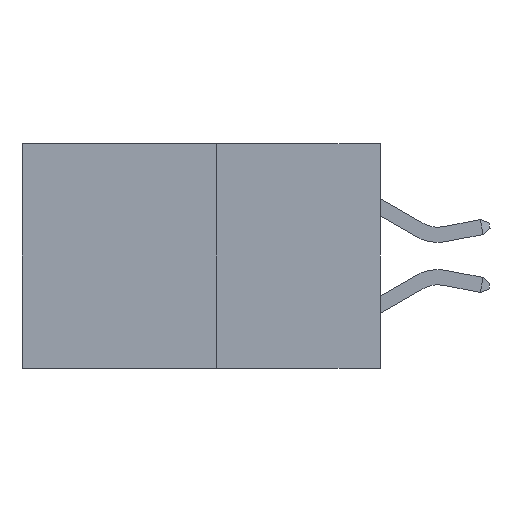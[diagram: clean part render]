
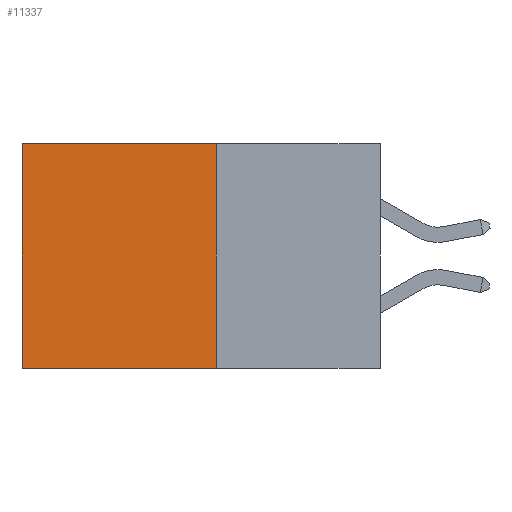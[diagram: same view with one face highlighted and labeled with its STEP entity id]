
A CAD part, left-side view. The second image highlights one B-rep face of the part: STEP entity #11337.
In plain terms, the highlighted planar face has unit normal (-1, 0, 0).
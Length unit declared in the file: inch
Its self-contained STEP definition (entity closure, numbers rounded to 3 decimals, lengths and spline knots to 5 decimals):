
#38 = CARTESIAN_POINT ( 'NONE',  ( 0.277, 0.27, -0.37 ) ) ;
#89 = LINE ( 'NONE', #1735, #9808 ) ;
#552 = DIRECTION ( 'NONE',  ( 0., 1., 0. ) ) ;
#641 = CARTESIAN_POINT ( 'NONE',  ( 0.277, 0.59, -0.37 ) ) ;
#710 = VECTOR ( 'NONE', #3658, 39.37008 ) ;
#1496 = CARTESIAN_POINT ( 'NONE',  ( 0.277, 0.59, -0.37 ) ) ;
#1546 = ORIENTED_EDGE ( 'NONE', *, *, #7881, .T. ) ;
#1735 = CARTESIAN_POINT ( 'NONE',  ( 0.277, 0.27, 0. ) ) ;
#2488 = VERTEX_POINT ( 'NONE', #1496 ) ;
#3043 = PLANE ( 'NONE',  #5065 ) ;
#3658 = DIRECTION ( 'NONE',  ( 0., 0., -1. ) ) ;
#3701 = LINE ( 'NONE', #3971, #8798 ) ;
#3971 = CARTESIAN_POINT ( 'NONE',  ( 0.277, 0.27, -0.37 ) ) ;
#4452 = EDGE_LOOP ( 'NONE', ( #6145, #6435, #11443, #1546 ) ) ;
#4520 = VERTEX_POINT ( 'NONE', #10834 ) ;
#4980 = DIRECTION ( 'NONE',  ( 0., 0., -1. ) ) ;
#5065 = AXIS2_PLACEMENT_3D ( 'NONE', #9770, #10687, #4980 ) ;
#5327 = EDGE_CURVE ( 'NONE', #9304, #7196, #3701, .T. ) ;
#5802 = EDGE_CURVE ( 'NONE', #4520, #2488, #8496, .T. ) ;
#6145 = ORIENTED_EDGE ( 'NONE', *, *, #5802, .T. ) ;
#6323 = LINE ( 'NONE', #6426, #11616 ) ;
#6426 = CARTESIAN_POINT ( 'NONE',  ( 0.277, 0.27, -0.37 ) ) ;
#6435 = ORIENTED_EDGE ( 'NONE', *, *, #9923, .F. ) ;
#7196 = VERTEX_POINT ( 'NONE', #38 ) ;
#7881 = EDGE_CURVE ( 'NONE', #9304, #4520, #89, .T. ) ;
#8496 = LINE ( 'NONE', #641, #710 ) ;
#8798 = VECTOR ( 'NONE', #10635, 39.37008 ) ;
#9304 = VERTEX_POINT ( 'NONE', #10520 ) ;
#9770 = CARTESIAN_POINT ( 'NONE',  ( 0.277, 0.27, -0.37 ) ) ;
#9808 = VECTOR ( 'NONE', #11295, 39.37008 ) ;
#9923 = EDGE_CURVE ( 'NONE', #7196, #2488, #6323, .T. ) ;
#10520 = CARTESIAN_POINT ( 'NONE',  ( 0.277, 0.27, 0. ) ) ;
#10614 = FACE_OUTER_BOUND ( 'NONE', #4452, .T. ) ;
#10635 = DIRECTION ( 'NONE',  ( 0., 0., -1. ) ) ;
#10687 = DIRECTION ( 'NONE',  ( 1., 0., 0. ) ) ;
#10834 = CARTESIAN_POINT ( 'NONE',  ( 0.277, 0.59, 0. ) ) ;
#11295 = DIRECTION ( 'NONE',  ( 0., 1., 0. ) ) ;
#11337 = ADVANCED_FACE ( 'NONE', ( #10614 ), #3043, .F. ) ;
#11443 = ORIENTED_EDGE ( 'NONE', *, *, #5327, .F. ) ;
#11616 = VECTOR ( 'NONE', #552, 39.37008 ) ;
